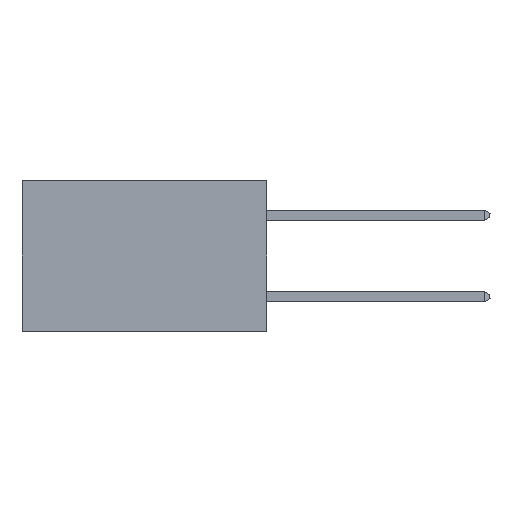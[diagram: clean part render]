
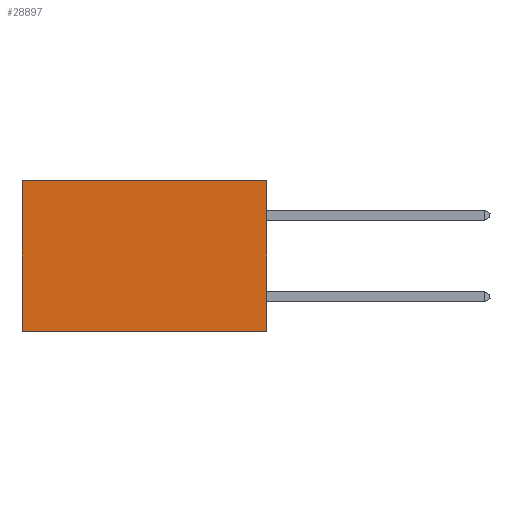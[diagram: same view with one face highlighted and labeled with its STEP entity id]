
A CAD part, left-side view. The second image highlights one B-rep face of the part: STEP entity #28897.
In plain terms, the highlighted planar face has unit normal (-1, 0, 0).
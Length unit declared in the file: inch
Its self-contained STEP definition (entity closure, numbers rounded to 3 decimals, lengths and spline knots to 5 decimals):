
#937 = EDGE_CURVE ( 'NONE', #33778, #13510, #19129, .T. ) ;
#1518 = CARTESIAN_POINT ( 'NONE',  ( 0.2875, 0.6, 0. ) ) ;
#1690 = CARTESIAN_POINT ( 'NONE',  ( 0.2875, 0., 0. ) ) ;
#3661 = CARTESIAN_POINT ( 'NONE',  ( 0.2875, 0.6, 0. ) ) ;
#5269 = DIRECTION ( 'NONE',  ( 0., 0., -1. ) ) ;
#5369 = EDGE_CURVE ( 'NONE', #13510, #31637, #32329, .T. ) ;
#6313 = DIRECTION ( 'NONE',  ( 0., 0., -1. ) ) ;
#9208 = VECTOR ( 'NONE', #12315, 39.37008 ) ;
#11661 = VECTOR ( 'NONE', #19646, 39.37008 ) ;
#11685 = AXIS2_PLACEMENT_3D ( 'NONE', #18431, #21069, #5269 ) ;
#11958 = EDGE_LOOP ( 'NONE', ( #26251, #27768, #19331, #24546 ) ) ;
#12315 = DIRECTION ( 'NONE',  ( 0., 1., 0. ) ) ;
#13510 = VERTEX_POINT ( 'NONE', #1518 ) ;
#17040 = EDGE_CURVE ( 'NONE', #33778, #23537, #22909, .T. ) ;
#18431 = CARTESIAN_POINT ( 'NONE',  ( 0.2875, 0., 0. ) ) ;
#19129 = LINE ( 'NONE', #30305, #9208 ) ;
#19331 = ORIENTED_EDGE ( 'NONE', *, *, #17040, .F. ) ;
#19636 = CARTESIAN_POINT ( 'NONE',  ( 0.2875, 0.6, -0.37 ) ) ;
#19646 = DIRECTION ( 'NONE',  ( 0., 1., 0. ) ) ;
#21069 = DIRECTION ( 'NONE',  ( 1., 0., 0. ) ) ;
#22909 = LINE ( 'NONE', #34011, #26199 ) ;
#23537 = VERTEX_POINT ( 'NONE', #26809 ) ;
#23620 = LINE ( 'NONE', #27473, #11661 ) ;
#23891 = DIRECTION ( 'NONE',  ( 0., 0., -1. ) ) ;
#24546 = ORIENTED_EDGE ( 'NONE', *, *, #937, .T. ) ;
#26199 = VECTOR ( 'NONE', #23891, 39.37008 ) ;
#26251 = ORIENTED_EDGE ( 'NONE', *, *, #5369, .T. ) ;
#26809 = CARTESIAN_POINT ( 'NONE',  ( 0.2875, 0., -0.37 ) ) ;
#27473 = CARTESIAN_POINT ( 'NONE',  ( 0.2875, 0., -0.37 ) ) ;
#27768 = ORIENTED_EDGE ( 'NONE', *, *, #32387, .F. ) ;
#28626 = PLANE ( 'NONE',  #11685 ) ;
#28897 = ADVANCED_FACE ( 'NONE', ( #29891 ), #28626, .F. ) ;
#29891 = FACE_OUTER_BOUND ( 'NONE', #11958, .T. ) ;
#30305 = CARTESIAN_POINT ( 'NONE',  ( 0.2875, 0., 0. ) ) ;
#31637 = VERTEX_POINT ( 'NONE', #19636 ) ;
#32329 = LINE ( 'NONE', #3661, #32705 ) ;
#32387 = EDGE_CURVE ( 'NONE', #23537, #31637, #23620, .T. ) ;
#32705 = VECTOR ( 'NONE', #6313, 39.37008 ) ;
#33778 = VERTEX_POINT ( 'NONE', #1690 ) ;
#34011 = CARTESIAN_POINT ( 'NONE',  ( 0.2875, 0., 0. ) ) ;
